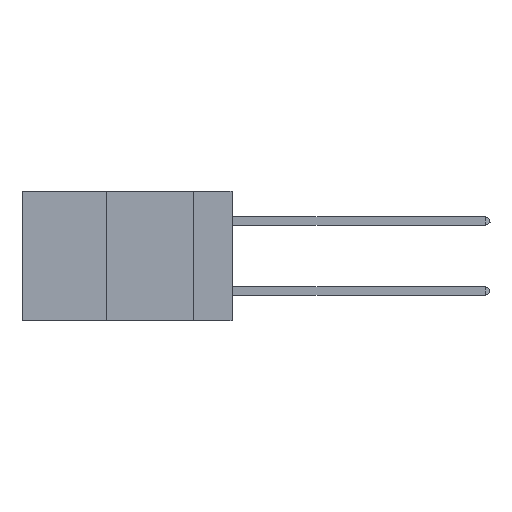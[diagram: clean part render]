
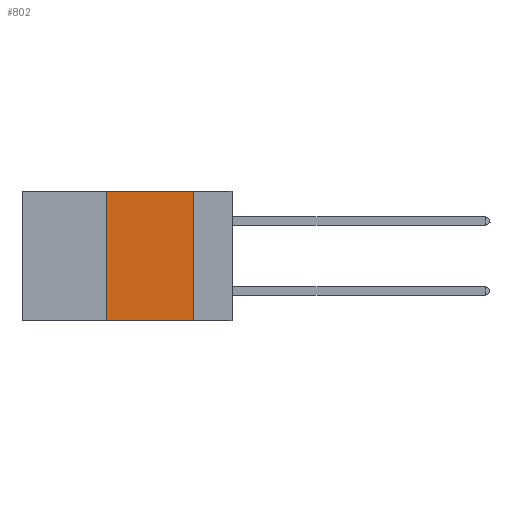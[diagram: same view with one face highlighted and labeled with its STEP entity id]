
A CAD part, left-side view. The second image highlights one B-rep face of the part: STEP entity #802.
In plain terms, the highlighted planar face has unit normal (-1, 0, 0).
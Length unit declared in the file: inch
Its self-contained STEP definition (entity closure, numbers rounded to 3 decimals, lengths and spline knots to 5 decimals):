
#247 = FACE_OUTER_BOUND ( 'NONE', #12171, .T. ) ;
#335 = CARTESIAN_POINT ( 'NONE',  ( 0., 0.6, -0.37 ) ) ;
#802 = ADVANCED_FACE ( 'NONE', ( #247 ), #5234, .F. ) ;
#1168 = EDGE_CURVE ( 'NONE', #5117, #2927, #4825, .T. ) ;
#1377 = ORIENTED_EDGE ( 'NONE', *, *, #2009, .F. ) ;
#2009 = EDGE_CURVE ( 'NONE', #2927, #5842, #10996, .T. ) ;
#2150 = EDGE_CURVE ( 'NONE', #7183, #5842, #10540, .T. ) ;
#2188 = CARTESIAN_POINT ( 'NONE',  ( 0., 0.36, 0. ) ) ;
#2449 = DIRECTION ( 'NONE',  ( 0., -1., 0. ) ) ;
#2927 = VERTEX_POINT ( 'NONE', #11004 ) ;
#3995 = ORIENTED_EDGE ( 'NONE', *, *, #1168, .F. ) ;
#4064 = VECTOR ( 'NONE', #2449, 39.37008 ) ;
#4315 = CARTESIAN_POINT ( 'NONE',  ( 0., 0.6, 0. ) ) ;
#4454 = CARTESIAN_POINT ( 'NONE',  ( 0., 0.11, -0.37 ) ) ;
#4825 = LINE ( 'NONE', #4315, #4064 ) ;
#4849 = CARTESIAN_POINT ( 'NONE',  ( 0., 0.11, 0. ) ) ;
#4855 = DIRECTION ( 'NONE',  ( 0., 0., -1. ) ) ;
#5117 = VERTEX_POINT ( 'NONE', #2188 ) ;
#5234 = PLANE ( 'NONE',  #11063 ) ;
#5531 = CARTESIAN_POINT ( 'NONE',  ( 0., 0.36, 0. ) ) ;
#5724 = ORIENTED_EDGE ( 'NONE', *, *, #2150, .T. ) ;
#5842 = VERTEX_POINT ( 'NONE', #4454 ) ;
#6601 = VECTOR ( 'NONE', #9353, 39.37008 ) ;
#7183 = VERTEX_POINT ( 'NONE', #11947 ) ;
#7605 = DIRECTION ( 'NONE',  ( 1., 0., 0. ) ) ;
#7718 = CARTESIAN_POINT ( 'NONE',  ( 0., 0.6, 0. ) ) ;
#8494 = VECTOR ( 'NONE', #11527, 39.37008 ) ;
#9353 = DIRECTION ( 'NONE',  ( 0., 0., 1. ) ) ;
#9704 = ORIENTED_EDGE ( 'NONE', *, *, #11782, .F. ) ;
#10409 = VECTOR ( 'NONE', #10766, 39.37008 ) ;
#10540 = LINE ( 'NONE', #335, #10409 ) ;
#10766 = DIRECTION ( 'NONE',  ( 0., -1., 0. ) ) ;
#10996 = LINE ( 'NONE', #4849, #8494 ) ;
#11004 = CARTESIAN_POINT ( 'NONE',  ( 0., 0.11, 0. ) ) ;
#11063 = AXIS2_PLACEMENT_3D ( 'NONE', #7718, #7605, #4855 ) ;
#11527 = DIRECTION ( 'NONE',  ( 0., 0., -1. ) ) ;
#11782 = EDGE_CURVE ( 'NONE', #7183, #5117, #11903, .T. ) ;
#11903 = LINE ( 'NONE', #5531, #6601 ) ;
#11947 = CARTESIAN_POINT ( 'NONE',  ( 0., 0.36, -0.37 ) ) ;
#12171 = EDGE_LOOP ( 'NONE', ( #1377, #3995, #9704, #5724 ) ) ;
